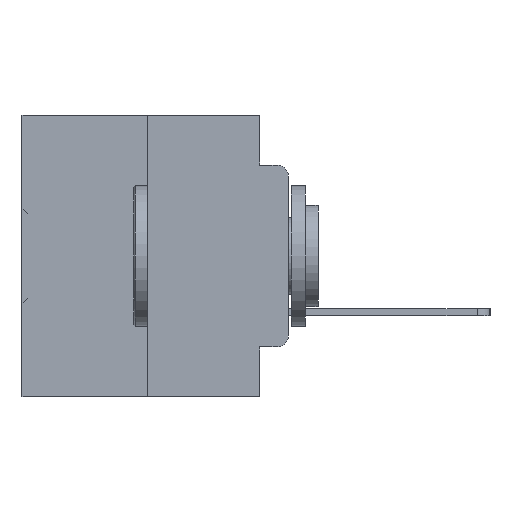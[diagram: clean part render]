
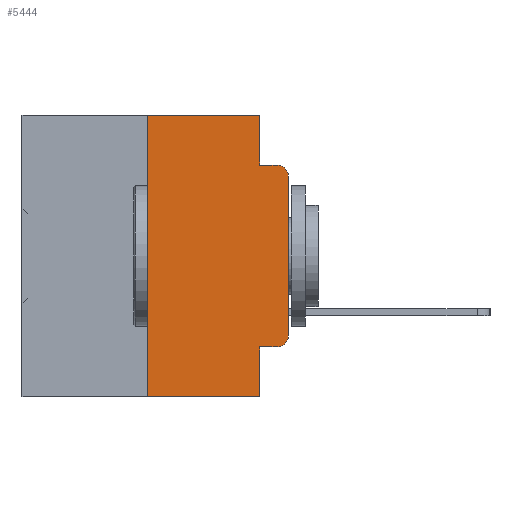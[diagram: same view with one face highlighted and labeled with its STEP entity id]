
A CAD part, left-side view. The second image highlights one B-rep face of the part: STEP entity #5444.
In plain terms, the highlighted planar face has unit normal (-1, 0, 0).
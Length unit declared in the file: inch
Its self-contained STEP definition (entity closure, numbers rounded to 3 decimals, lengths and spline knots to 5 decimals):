
#63 = ORIENTED_EDGE ( 'NONE', *, *, #30930, .T. ) ;
#682 = DIRECTION ( 'NONE',  ( -1., 0., 0. ) ) ;
#1521 = LINE ( 'NONE', #32309, #31537 ) ;
#1818 = CARTESIAN_POINT ( 'NONE',  ( 0., 0.02, -0.1085 ) ) ;
#1836 = VECTOR ( 'NONE', #3656, 39.37008 ) ;
#2138 = LINE ( 'NONE', #8391, #19595 ) ;
#3107 = CARTESIAN_POINT ( 'NONE',  ( 0., 0.051, -0.4115 ) ) ;
#3656 = DIRECTION ( 'NONE',  ( 0., 0., 1. ) ) ;
#4725 = VERTEX_POINT ( 'NONE', #21770 ) ;
#4841 = DIRECTION ( 'NONE',  ( 0., 0., -1. ) ) ;
#5045 = CARTESIAN_POINT ( 'NONE',  ( 0., 0.051, 0. ) ) ;
#5158 = DIRECTION ( 'NONE',  ( 1., 0., 0. ) ) ;
#5444 = ADVANCED_FACE ( 'NONE', ( #8366 ), #22631, .F. ) ;
#6019 = EDGE_CURVE ( 'NONE', #10407, #13715, #35866, .T. ) ;
#6146 = ORIENTED_EDGE ( 'NONE', *, *, #21485, .F. ) ;
#6554 = CARTESIAN_POINT ( 'NONE',  ( 0., 0.25, -0.5 ) ) ;
#7064 = ORIENTED_EDGE ( 'NONE', *, *, #24946, .F. ) ;
#7205 = EDGE_CURVE ( 'NONE', #18320, #4725, #2138, .T. ) ;
#7253 = CARTESIAN_POINT ( 'NONE',  ( 0., 0., 0. ) ) ;
#8323 = CARTESIAN_POINT ( 'NONE',  ( 0., 0.051, -0.0885 ) ) ;
#8366 = FACE_OUTER_BOUND ( 'NONE', #23373, .T. ) ;
#8391 = CARTESIAN_POINT ( 'NONE',  ( 0., 0.051, -0.4115 ) ) ;
#8415 = ORIENTED_EDGE ( 'NONE', *, *, #29283, .T. ) ;
#9495 = VECTOR ( 'NONE', #25446, 39.37008 ) ;
#10369 = AXIS2_PLACEMENT_3D ( 'NONE', #16822, #5158, #25548 ) ;
#10407 = VERTEX_POINT ( 'NONE', #8323 ) ;
#10993 = CARTESIAN_POINT ( 'NONE',  ( 0., 0.25, 0. ) ) ;
#11091 = VECTOR ( 'NONE', #11584, 39.37008 ) ;
#11584 = DIRECTION ( 'NONE',  ( 0., -1., 0. ) ) ;
#11781 = CARTESIAN_POINT ( 'NONE',  ( 0., 0., -0.1085 ) ) ;
#12141 = DIRECTION ( 'NONE',  ( 0., -1., 0. ) ) ;
#13715 = VERTEX_POINT ( 'NONE', #33203 ) ;
#13818 = VECTOR ( 'NONE', #24355, 39.37008 ) ;
#14208 = LINE ( 'NONE', #7253, #15129 ) ;
#14733 = LINE ( 'NONE', #35756, #13818 ) ;
#15076 = EDGE_CURVE ( 'NONE', #18319, #10407, #17299, .T. ) ;
#15129 = VECTOR ( 'NONE', #24694, 39.37008 ) ;
#15362 = CARTESIAN_POINT ( 'NONE',  ( 0., 0.25, 0. ) ) ;
#16004 = EDGE_CURVE ( 'NONE', #4725, #18865, #33368, .T. ) ;
#16822 = CARTESIAN_POINT ( 'NONE',  ( 0., 0.473, 0. ) ) ;
#16928 = CARTESIAN_POINT ( 'NONE',  ( 0., 0.051, -0.5 ) ) ;
#17299 = LINE ( 'NONE', #5045, #9495 ) ;
#17474 = VERTEX_POINT ( 'NONE', #10993 ) ;
#18029 = ORIENTED_EDGE ( 'NONE', *, *, #15076, .F. ) ;
#18296 = CARTESIAN_POINT ( 'NONE',  ( 0., 0.02, -0.3915 ) ) ;
#18319 = VERTEX_POINT ( 'NONE', #20645 ) ;
#18320 = VERTEX_POINT ( 'NONE', #3107 ) ;
#18865 = VERTEX_POINT ( 'NONE', #35511 ) ;
#18905 = LINE ( 'NONE', #31803, #11091 ) ;
#19304 = LINE ( 'NONE', #15362, #1836 ) ;
#19595 = VECTOR ( 'NONE', #28660, 39.37008 ) ;
#20645 = CARTESIAN_POINT ( 'NONE',  ( 0., 0.051, 0. ) ) ;
#20655 = AXIS2_PLACEMENT_3D ( 'NONE', #18296, #682, #21190 ) ;
#20681 = VECTOR ( 'NONE', #30959, 39.37008 ) ;
#21190 = DIRECTION ( 'NONE',  ( 0., 0., -1. ) ) ;
#21485 = EDGE_CURVE ( 'NONE', #17474, #18319, #1521, .T. ) ;
#21770 = CARTESIAN_POINT ( 'NONE',  ( 0., 0.02, -0.4115 ) ) ;
#22319 = DIRECTION ( 'NONE',  ( -1., 0., 0. ) ) ;
#22631 = PLANE ( 'NONE',  #10369 ) ;
#22652 = VERTEX_POINT ( 'NONE', #11781 ) ;
#23001 = ORIENTED_EDGE ( 'NONE', *, *, #25724, .T. ) ;
#23129 = VERTEX_POINT ( 'NONE', #16928 ) ;
#23373 = EDGE_LOOP ( 'NONE', ( #23001, #8415, #32355, #18029, #6146, #7064, #63, #26183, #27953, #30650 ) ) ;
#24355 = DIRECTION ( 'NONE',  ( 0., 0., -1. ) ) ;
#24694 = DIRECTION ( 'NONE',  ( 0., 0., 1. ) ) ;
#24946 = EDGE_CURVE ( 'NONE', #33774, #17474, #19304, .T. ) ;
#25049 = EDGE_CURVE ( 'NONE', #18320, #23129, #14733, .T. ) ;
#25258 = CARTESIAN_POINT ( 'NONE',  ( 0., 0.051, -0.0885 ) ) ;
#25446 = DIRECTION ( 'NONE',  ( 0., 0., -1. ) ) ;
#25548 = DIRECTION ( 'NONE',  ( 0., 0., -1. ) ) ;
#25724 = EDGE_CURVE ( 'NONE', #18865, #22652, #14208, .T. ) ;
#26183 = ORIENTED_EDGE ( 'NONE', *, *, #25049, .F. ) ;
#27953 = ORIENTED_EDGE ( 'NONE', *, *, #7205, .T. ) ;
#28660 = DIRECTION ( 'NONE',  ( 0., -1., 0. ) ) ;
#29283 = EDGE_CURVE ( 'NONE', #22652, #13715, #33319, .T. ) ;
#30650 = ORIENTED_EDGE ( 'NONE', *, *, #16004, .T. ) ;
#30930 = EDGE_CURVE ( 'NONE', #33774, #23129, #18905, .T. ) ;
#30959 = DIRECTION ( 'NONE',  ( 0., -1., 0. ) ) ;
#31537 = VECTOR ( 'NONE', #12141, 39.37008 ) ;
#31769 = AXIS2_PLACEMENT_3D ( 'NONE', #1818, #22319, #4841 ) ;
#31803 = CARTESIAN_POINT ( 'NONE',  ( 0., 0.473, -0.5 ) ) ;
#32309 = CARTESIAN_POINT ( 'NONE',  ( 0., 0.473, 0. ) ) ;
#32355 = ORIENTED_EDGE ( 'NONE', *, *, #6019, .F. ) ;
#33203 = CARTESIAN_POINT ( 'NONE',  ( 0., 0.02, -0.0885 ) ) ;
#33319 = CIRCLE ( 'NONE', #31769, 0.02 ) ;
#33368 = CIRCLE ( 'NONE', #20655, 0.02 ) ;
#33774 = VERTEX_POINT ( 'NONE', #6554 ) ;
#35511 = CARTESIAN_POINT ( 'NONE',  ( 0., 0., -0.3915 ) ) ;
#35756 = CARTESIAN_POINT ( 'NONE',  ( 0., 0.051, 0. ) ) ;
#35866 = LINE ( 'NONE', #25258, #20681 ) ;
